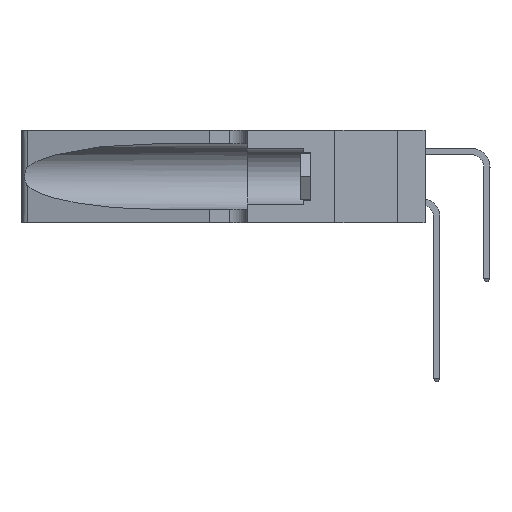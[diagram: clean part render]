
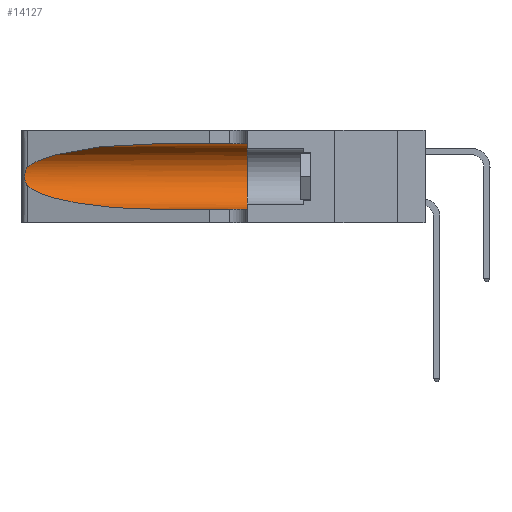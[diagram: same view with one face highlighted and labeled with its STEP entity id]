
A CAD part, left-side view. The second image highlights one B-rep face of the part: STEP entity #14127.
In plain terms, the highlighted cylindrical face has radius 3.308 mm (diameter 6.617 mm), a partial arc.
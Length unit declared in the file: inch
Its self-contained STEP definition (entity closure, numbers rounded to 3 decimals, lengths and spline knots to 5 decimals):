
#1096 = B_SPLINE_CURVE_WITH_KNOTS ( 'NONE', 3,
 ( #18107, #10627, #34601, #11788, #23747, #29256, #20479, #2438, #35522, #23487, #30135, #17826, #18203, #9248 ),
 .UNSPECIFIED., .F., .F.,
 ( 4, 2, 2, 2, 2, 2, 4 ),
 ( 0., 0.00027, 0.00053, 0.00107, 0.0016, 0.00187, 0.00214 ),
 .UNSPECIFIED. ) ;
#1536 = EDGE_CURVE ( 'NONE', #18119, #17892, #20887, .T. ) ;
#1624 = ORIENTED_EDGE ( 'NONE', *, *, #31259, .T. ) ;
#2438 = CARTESIAN_POINT ( 'NONE',  ( 0.26075, 1.23896, 0.178 ) ) ;
#2516 = VECTOR ( 'NONE', #18291, 39.37008 ) ;
#2720 = AXIS2_PLACEMENT_3D ( 'NONE', #27821, #36149, #22447 ) ;
#2822 = ORIENTED_EDGE ( 'NONE', *, *, #12712, .T. ) ;
#7289 = CARTESIAN_POINT ( 'NONE',  ( 0.25487, 1.22718, 0.22369 ) ) ;
#7426 = ORIENTED_EDGE ( 'NONE', *, *, #10121, .F. ) ;
#8788 = DIRECTION ( 'NONE',  ( 0., -1., 0. ) ) ;
#9248 = CARTESIAN_POINT ( 'NONE',  ( 0.25487, 1.22718, 0.14631 ) ) ;
#9738 =( BOUNDED_CURVE ( )  B_SPLINE_CURVE ( 3, ( #25286, #24895, #31297, #13386 ),
 .UNSPECIFIED., .F., .F. ) 
 B_SPLINE_CURVE_WITH_KNOTS ( ( 4, 4 ),
 ( 1.5708, 2.84003 ),
 .UNSPECIFIED. ) 
 CURVE ( )  GEOMETRIC_REPRESENTATION_ITEM ( )  RATIONAL_B_SPLINE_CURVE ( ( 1., 0.87, 0.87, 1. ) ) 
 REPRESENTATION_ITEM ( '' )  );
#10121 = EDGE_CURVE ( 'NONE', #17892, #38016, #28450, .T. ) ;
#10496 = VERTEX_POINT ( 'NONE', #23061 ) ;
#10627 = CARTESIAN_POINT ( 'NONE',  ( 0.25555, 1.22994, 0.2215 ) ) ;
#11788 = CARTESIAN_POINT ( 'NONE',  ( 0.25787, 1.23484, 0.2124 ) ) ;
#12712 = EDGE_CURVE ( 'NONE', #37268, #24777, #1096, .T. ) ;
#13386 = CARTESIAN_POINT ( 'NONE',  ( 0.25487, 1.22718, 0.22369 ) ) ;
#13780 = EDGE_CURVE ( 'NONE', #10496, #38016, #27300, .T. ) ;
#14127 = ADVANCED_FACE ( 'NONE', ( #21646 ), #22616, .F. ) ;
#16568 = ORIENTED_EDGE ( 'NONE', *, *, #13780, .T. ) ;
#17826 = CARTESIAN_POINT ( 'NONE',  ( 0.25639, 1.23186, 0.15144 ) ) ;
#17892 = VERTEX_POINT ( 'NONE', #22088 ) ;
#18107 = CARTESIAN_POINT ( 'NONE',  ( 0.25487, 1.22718, 0.22369 ) ) ;
#18119 = VERTEX_POINT ( 'NONE', #23759 ) ;
#18203 = CARTESIAN_POINT ( 'NONE',  ( 0.25555, 1.22993, 0.14849 ) ) ;
#18291 = DIRECTION ( 'NONE',  ( 0., -1., 0. ) ) ;
#18815 = ORIENTED_EDGE ( 'NONE', *, *, #24838, .T. ) ;
#18825 = CARTESIAN_POINT ( 'NONE',  ( 0.1305, 1.61858, 0.05475 ) ) ;
#19962 = CARTESIAN_POINT ( 'NONE',  ( 0.25487, 1.22718, 0.14631 ) ) ;
#20479 = CARTESIAN_POINT ( 'NONE',  ( 0.26075, 1.23896, 0.19203 ) ) ;
#20585 = CARTESIAN_POINT ( 'NONE',  ( 0.1305, 0.35, 0.05475 ) ) ;
#20887 = LINE ( 'NONE', #27433, #2516 ) ;
#21646 = FACE_OUTER_BOUND ( 'NONE', #27283, .T. ) ;
#21684 = VECTOR ( 'NONE', #30975, 39.37008 ) ;
#22088 = CARTESIAN_POINT ( 'NONE',  ( 0.1305, 0.35, 0.31525 ) ) ;
#22447 = DIRECTION ( 'NONE',  ( 0., 0., 1. ) ) ;
#22616 = CYLINDRICAL_SURFACE ( 'NONE', #38792, 0.13025 ) ;
#23061 = CARTESIAN_POINT ( 'NONE',  ( 0.1305, 0.72297, 0.05475 ) ) ;
#23419 = CARTESIAN_POINT ( 'NONE',  ( 0.2373, 1.15595, 0.08982 ) ) ;
#23487 = CARTESIAN_POINT ( 'NONE',  ( 0.25856, 1.23593, 0.16098 ) ) ;
#23747 = CARTESIAN_POINT ( 'NONE',  ( 0.25854, 1.2359, 0.20912 ) ) ;
#23759 = CARTESIAN_POINT ( 'NONE',  ( 0.1305, 0.72297, 0.31525 ) ) ;
#24413 =( BOUNDED_CURVE ( )  B_SPLINE_CURVE ( 3, ( #32668, #23419, #38480, #29568 ),
 .UNSPECIFIED., .F., .F. ) 
 B_SPLINE_CURVE_WITH_KNOTS ( ( 4, 4 ),
 ( 3.44316, 4.71239 ),
 .UNSPECIFIED. ) 
 CURVE ( )  GEOMETRIC_REPRESENTATION_ITEM ( )  RATIONAL_B_SPLINE_CURVE ( ( 1., 0.87, 0.87, 1. ) ) 
 REPRESENTATION_ITEM ( '' )  );
#24777 = VERTEX_POINT ( 'NONE', #19962 ) ;
#24838 = EDGE_CURVE ( 'NONE', #24777, #10496, #24413, .T. ) ;
#24895 = CARTESIAN_POINT ( 'NONE',  ( 0.18966, 0.96281, 0.31525 ) ) ;
#25286 = CARTESIAN_POINT ( 'NONE',  ( 0.1305, 0.72297, 0.31525 ) ) ;
#26756 = CARTESIAN_POINT ( 'NONE',  ( 0.1305, 1.61858, 0.185 ) ) ;
#27283 = EDGE_LOOP ( 'NONE', ( #1624, #2822, #18815, #16568, #7426, #36696 ) ) ;
#27300 = LINE ( 'NONE', #18825, #21684 ) ;
#27433 = CARTESIAN_POINT ( 'NONE',  ( 0.1305, 1.61858, 0.31525 ) ) ;
#27821 = CARTESIAN_POINT ( 'NONE',  ( 0.1305, 0.35, 0.185 ) ) ;
#28450 = CIRCLE ( 'NONE', #2720, 0.13025 ) ;
#29256 = CARTESIAN_POINT ( 'NONE',  ( 0.26018, 1.23835, 0.19895 ) ) ;
#29568 = CARTESIAN_POINT ( 'NONE',  ( 0.1305, 0.72297, 0.05475 ) ) ;
#30135 = CARTESIAN_POINT ( 'NONE',  ( 0.25789, 1.23486, 0.15765 ) ) ;
#30975 = DIRECTION ( 'NONE',  ( 0., -1., 0. ) ) ;
#31259 = EDGE_CURVE ( 'NONE', #18119, #37268, #9738, .T. ) ;
#31297 = CARTESIAN_POINT ( 'NONE',  ( 0.2373, 1.15595, 0.28018 ) ) ;
#32236 = DIRECTION ( 'NONE',  ( 0., 0., -1. ) ) ;
#32668 = CARTESIAN_POINT ( 'NONE',  ( 0.25487, 1.22718, 0.14631 ) ) ;
#34601 = CARTESIAN_POINT ( 'NONE',  ( 0.25639, 1.23184, 0.21858 ) ) ;
#35522 = CARTESIAN_POINT ( 'NONE',  ( 0.26017, 1.23833, 0.17102 ) ) ;
#36149 = DIRECTION ( 'NONE',  ( 0., 1., 0. ) ) ;
#36696 = ORIENTED_EDGE ( 'NONE', *, *, #1536, .F. ) ;
#37268 = VERTEX_POINT ( 'NONE', #7289 ) ;
#38016 = VERTEX_POINT ( 'NONE', #20585 ) ;
#38480 = CARTESIAN_POINT ( 'NONE',  ( 0.18966, 0.96281, 0.05475 ) ) ;
#38792 = AXIS2_PLACEMENT_3D ( 'NONE', #26756, #8788, #32236 ) ;
